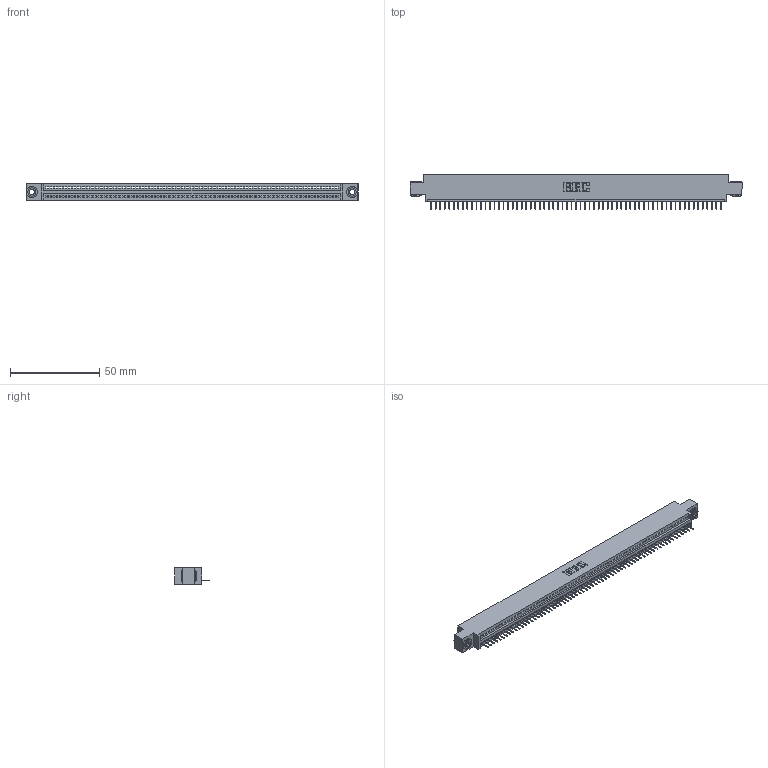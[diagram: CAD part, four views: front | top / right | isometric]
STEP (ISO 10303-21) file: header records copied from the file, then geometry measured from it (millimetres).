
FILE_DESCRIPTION (( 'STEP AP203' ), '1' );
FILE_NAME ('345-065-524-603.STEP', '2018-09-28T13:35:28', ( '' ), ( '' ), 'SwSTEP 2.0', 'SolidWorks 2016', '' );
FILE_SCHEMA (( 'CONFIG_CONTROL_DESIGN' ));
Length unit declared in the file: inch
Products named in the file (4): 345-065-524-603; 345 Part_0.170 Offset - 0.156 Dia-TH; 345-250-002_345-250-002-102; 345-292-001_345-293-124
Assembly tree (68 placements, depth 2):
  345-065-524-603
    345 Part_0.170 Offset - 0.156 Dia-TH
    345-292-001_345-293-124  x65
    345-250-002_345-250-002-102  x2
Bounding box: 186.31 x 19.35 x 9.4 mm (x, y, z)
Volume: 17533.5 mm3; surface area: 23133 mm2
Topology: 68 solids, 68 shells, 4198 faces, 12129 edges, 7822 vertices
Faces by surface type: plane 3084, cylinder 1106, cone 8
Entity records: 46680 total; most frequent: CARTESIAN_POINT 8062, ORIENTED_EDGE 8054, DIRECTION 7039, EDGE_CURVE 4027, VECTOR 3615, LINE 3615, VERTEX_POINT 2678, AXIS2_PLACEMENT_3D 1712
